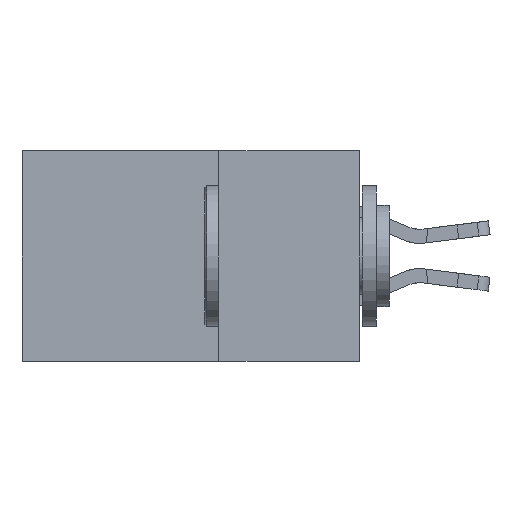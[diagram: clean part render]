
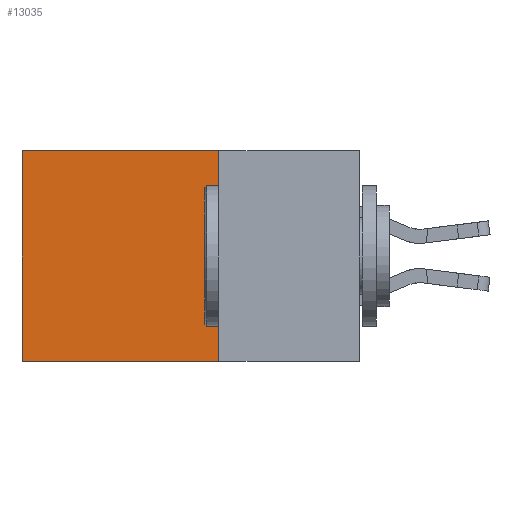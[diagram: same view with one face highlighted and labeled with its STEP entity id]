
A CAD part, left-side view. The second image highlights one B-rep face of the part: STEP entity #13035.
In plain terms, the highlighted planar face has unit normal (-1, 0, 0).
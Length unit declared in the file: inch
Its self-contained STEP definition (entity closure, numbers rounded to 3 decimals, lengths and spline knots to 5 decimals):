
#41 = ORIENTED_EDGE ( 'NONE', *, *, #13892, .T. ) ;
#168 = VERTEX_POINT ( 'NONE', #2310 ) ;
#291 = ORIENTED_EDGE ( 'NONE', *, *, #2215, .F. ) ;
#353 = CARTESIAN_POINT ( 'NONE',  ( 0.2875, 0.6, 0. ) ) ;
#756 = DIRECTION ( 'NONE',  ( 1., 0., 0. ) ) ;
#837 = FACE_OUTER_BOUND ( 'NONE', #14406, .T. ) ;
#1539 = VECTOR ( 'NONE', #10168, 39.37008 ) ;
#1676 = LINE ( 'NONE', #6143, #7864 ) ;
#2013 = EDGE_CURVE ( 'NONE', #168, #4984, #3547, .T. ) ;
#2215 = EDGE_CURVE ( 'NONE', #4984, #4869, #8666, .T. ) ;
#2310 = CARTESIAN_POINT ( 'NONE',  ( 0.2875, 0.25, 0. ) ) ;
#2524 = ORIENTED_EDGE ( 'NONE', *, *, #9382, .T. ) ;
#3092 = DIRECTION ( 'NONE',  ( 0., 1., 0. ) ) ;
#3547 = LINE ( 'NONE', #13576, #1539 ) ;
#3601 = CARTESIAN_POINT ( 'NONE',  ( 0.2875, 0.6, -0.375 ) ) ;
#4869 = VERTEX_POINT ( 'NONE', #5413 ) ;
#4984 = VERTEX_POINT ( 'NONE', #8144 ) ;
#5413 = CARTESIAN_POINT ( 'NONE',  ( 0.2875, 0.6, -0.375 ) ) ;
#5818 = VECTOR ( 'NONE', #3092, 39.37008 ) ;
#6143 = CARTESIAN_POINT ( 'NONE',  ( 0.2875, 0.25, 0. ) ) ;
#6194 = PLANE ( 'NONE',  #11478 ) ;
#7864 = VECTOR ( 'NONE', #9476, 39.37008 ) ;
#8144 = CARTESIAN_POINT ( 'NONE',  ( 0.2875, 0.25, -0.375 ) ) ;
#8173 = VECTOR ( 'NONE', #11345, 39.37008 ) ;
#8540 = ORIENTED_EDGE ( 'NONE', *, *, #2013, .F. ) ;
#8666 = LINE ( 'NONE', #12080, #5818 ) ;
#9207 = VERTEX_POINT ( 'NONE', #353 ) ;
#9382 = EDGE_CURVE ( 'NONE', #9207, #4869, #13638, .T. ) ;
#9476 = DIRECTION ( 'NONE',  ( 0., 1., 0. ) ) ;
#9753 = CARTESIAN_POINT ( 'NONE',  ( 0.2875, 0.25, -0.375 ) ) ;
#10168 = DIRECTION ( 'NONE',  ( 0., 0., -1. ) ) ;
#11345 = DIRECTION ( 'NONE',  ( 0., 0., -1. ) ) ;
#11478 = AXIS2_PLACEMENT_3D ( 'NONE', #9753, #756, #14063 ) ;
#12080 = CARTESIAN_POINT ( 'NONE',  ( 0.2875, 0.25, -0.375 ) ) ;
#13035 = ADVANCED_FACE ( 'NONE', ( #837 ), #6194, .F. ) ;
#13576 = CARTESIAN_POINT ( 'NONE',  ( 0.2875, 0.25, -0.375 ) ) ;
#13638 = LINE ( 'NONE', #3601, #8173 ) ;
#13892 = EDGE_CURVE ( 'NONE', #168, #9207, #1676, .T. ) ;
#14063 = DIRECTION ( 'NONE',  ( 0., 0., -1. ) ) ;
#14406 = EDGE_LOOP ( 'NONE', ( #2524, #291, #8540, #41 ) ) ;
